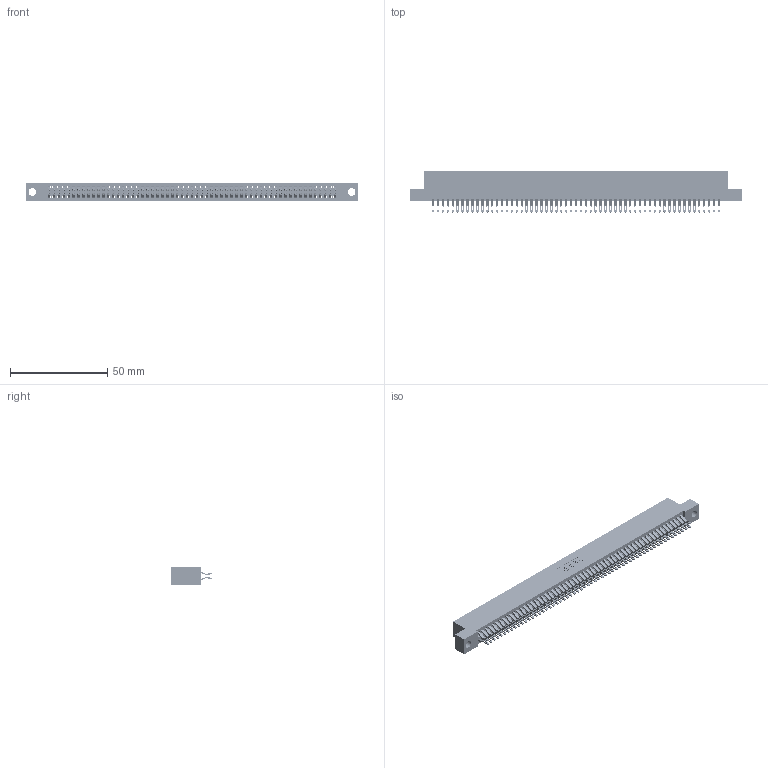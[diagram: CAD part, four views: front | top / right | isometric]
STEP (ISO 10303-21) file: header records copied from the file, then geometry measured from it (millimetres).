
FILE_DESCRIPTION (( 'STEP AP203' ), '1' );
FILE_NAME ('845-118-555-204.STEP', '2018-11-20T21:56:58', ( '' ), ( '' ), 'SwSTEP 2.0', 'SolidWorks 2016', '' );
FILE_SCHEMA (( 'CONFIG_CONTROL_DESIGN' ));
Length unit declared in the file: inch
Products named in the file (3): 845 Part_Flush Mounting Lugs - 0.156 Dia-TH; 345-292-001_555 Tail; 845-118-555-204
Assembly tree (119 placements, depth 2):
  845-118-555-204
    845 Part_Flush Mounting Lugs - 0.156 Dia-TH
    345-292-001_555 Tail  x118
Bounding box: 171.07 x 21.13 x 9.4 mm (x, y, z)
Volume: 17030 mm3; surface area: 26508.1 mm2
Topology: 119 solids, 119 shells, 6734 faces, 21227 edges, 14150 vertices
Faces by surface type: plane 3738, cylinder 2996
Entity records: 44333 total; most frequent: CARTESIAN_POINT 7450, ORIENTED_EDGE 7354, DIRECTION 6517, EDGE_CURVE 3677, LINE 3289, VECTOR 3289, VERTEX_POINT 2450, AXIS2_PLACEMENT_3D 1614
